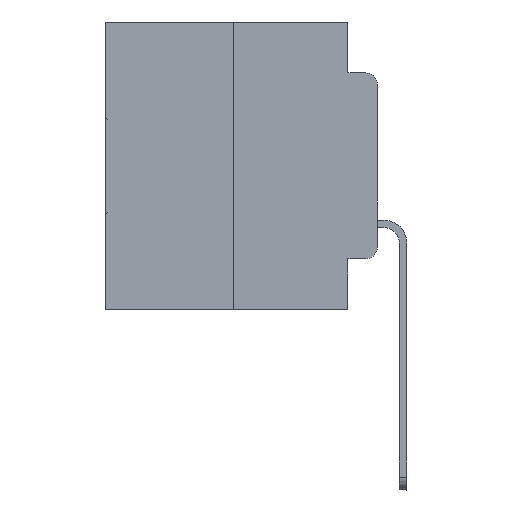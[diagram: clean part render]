
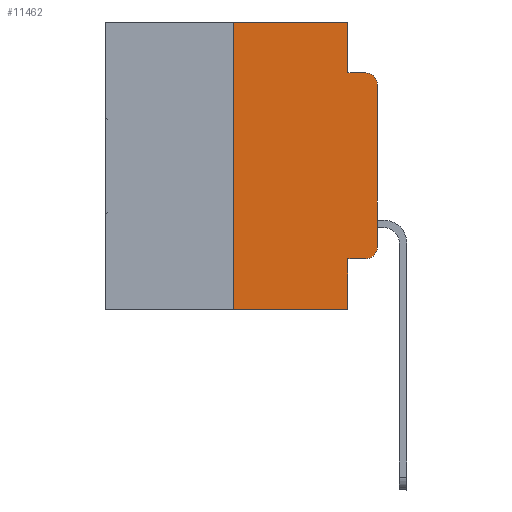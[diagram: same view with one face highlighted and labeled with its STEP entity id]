
A CAD part, left-side view. The second image highlights one B-rep face of the part: STEP entity #11462.
In plain terms, the highlighted planar face has unit normal (-1, 0, 0).
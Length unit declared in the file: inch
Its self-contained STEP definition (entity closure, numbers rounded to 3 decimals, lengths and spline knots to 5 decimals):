
#72 = CARTESIAN_POINT ( 'NONE',  ( 0., 0.051, 0. ) ) ;
#198 = VECTOR ( 'NONE', #6919, 39.37008 ) ;
#233 = CARTESIAN_POINT ( 'NONE',  ( 0., 0.02, -0.1085 ) ) ;
#1229 = VECTOR ( 'NONE', #27164, 39.37008 ) ;
#1791 = LINE ( 'NONE', #11337, #1229 ) ;
#2072 = CARTESIAN_POINT ( 'NONE',  ( 0., 0., 0. ) ) ;
#2083 = VECTOR ( 'NONE', #19083, 39.37008 ) ;
#2942 = LINE ( 'NONE', #9962, #2083 ) ;
#2987 = DIRECTION ( 'NONE',  ( 1., 0., 0. ) ) ;
#3520 = VECTOR ( 'NONE', #17909, 39.37008 ) ;
#4189 = ORIENTED_EDGE ( 'NONE', *, *, #8577, .F. ) ;
#4339 = ORIENTED_EDGE ( 'NONE', *, *, #24047, .F. ) ;
#4835 = LINE ( 'NONE', #24819, #198 ) ;
#5237 = DIRECTION ( 'NONE',  ( 0., 0., -1. ) ) ;
#5364 = VERTEX_POINT ( 'NONE', #17767 ) ;
#5476 = CARTESIAN_POINT ( 'NONE',  ( 0., 0.051, 0. ) ) ;
#6383 = ORIENTED_EDGE ( 'NONE', *, *, #21122, .T. ) ;
#6919 = DIRECTION ( 'NONE',  ( 0., 0., 1. ) ) ;
#8302 = LINE ( 'NONE', #5476, #18983 ) ;
#8577 = EDGE_CURVE ( 'NONE', #17255, #16914, #2942, .T. ) ;
#8653 = DIRECTION ( 'NONE',  ( 0., 0., 1. ) ) ;
#8790 = LINE ( 'NONE', #29236, #3520 ) ;
#8833 = EDGE_CURVE ( 'NONE', #5364, #15069, #4835, .T. ) ;
#9390 = DIRECTION ( 'NONE',  ( 0., 0., -1. ) ) ;
#9706 = EDGE_CURVE ( 'NONE', #5364, #25665, #8790, .T. ) ;
#9962 = CARTESIAN_POINT ( 'NONE',  ( 0., 0.051, -0.0885 ) ) ;
#10247 = CARTESIAN_POINT ( 'NONE',  ( 0., 0., -0.3915 ) ) ;
#11337 = CARTESIAN_POINT ( 'NONE',  ( 0., 0.051, -0.4115 ) ) ;
#11462 = ADVANCED_FACE ( 'NONE', ( #21215 ), #16591, .F. ) ;
#11652 = ORIENTED_EDGE ( 'NONE', *, *, #8833, .F. ) ;
#11819 = ORIENTED_EDGE ( 'NONE', *, *, #9706, .T. ) ;
#12499 = DIRECTION ( 'NONE',  ( 0., 0., -1. ) ) ;
#12764 = CARTESIAN_POINT ( 'NONE',  ( 0., 0.02, -0.0885 ) ) ;
#12994 = LINE ( 'NONE', #2072, #23871 ) ;
#13425 = EDGE_CURVE ( 'NONE', #22376, #20475, #21812, .T. ) ;
#13548 = DIRECTION ( 'NONE',  ( 0., 0., -1. ) ) ;
#13746 = CARTESIAN_POINT ( 'NONE',  ( 0., 0.051, 0. ) ) ;
#14175 = VECTOR ( 'NONE', #9390, 39.37008 ) ;
#15069 = VERTEX_POINT ( 'NONE', #25286 ) ;
#15213 = EDGE_CURVE ( 'NONE', #23148, #17255, #8302, .T. ) ;
#15315 = VECTOR ( 'NONE', #27217, 39.37008 ) ;
#15753 = CARTESIAN_POINT ( 'NONE',  ( 0., 0.473, 0. ) ) ;
#16043 = CARTESIAN_POINT ( 'NONE',  ( 0., 0.051, -0.0885 ) ) ;
#16382 = DIRECTION ( 'NONE',  ( 0., 0., -1. ) ) ;
#16591 = PLANE ( 'NONE',  #19329 ) ;
#16650 = AXIS2_PLACEMENT_3D ( 'NONE', #233, #18336, #16382 ) ;
#16914 = VERTEX_POINT ( 'NONE', #12764 ) ;
#16941 = ORIENTED_EDGE ( 'NONE', *, *, #18420, .F. ) ;
#17255 = VERTEX_POINT ( 'NONE', #16043 ) ;
#17767 = CARTESIAN_POINT ( 'NONE',  ( 0., 0.25, -0.5 ) ) ;
#17909 = DIRECTION ( 'NONE',  ( 0., -1., 0. ) ) ;
#18336 = DIRECTION ( 'NONE',  ( -1., 0., 0. ) ) ;
#18348 = EDGE_LOOP ( 'NONE', ( #28187, #28456, #4189, #22299, #16941, #11652, #11819, #4339, #6383, #21950 ) ) ;
#18420 = EDGE_CURVE ( 'NONE', #15069, #23148, #22760, .T. ) ;
#18475 = CARTESIAN_POINT ( 'NONE',  ( 0., 0.02, -0.3915 ) ) ;
#18634 = CARTESIAN_POINT ( 'NONE',  ( 0., 0.051, -0.5 ) ) ;
#18845 = CARTESIAN_POINT ( 'NONE',  ( 0., 0., -0.1085 ) ) ;
#18983 = VECTOR ( 'NONE', #12499, 39.37008 ) ;
#19007 = VERTEX_POINT ( 'NONE', #18845 ) ;
#19083 = DIRECTION ( 'NONE',  ( 0., -1., 0. ) ) ;
#19129 = CARTESIAN_POINT ( 'NONE',  ( 0., 0.473, 0. ) ) ;
#19329 = AXIS2_PLACEMENT_3D ( 'NONE', #19129, #2987, #5237 ) ;
#19928 = CARTESIAN_POINT ( 'NONE',  ( 0., 0.02, -0.4115 ) ) ;
#20185 = VERTEX_POINT ( 'NONE', #29521 ) ;
#20475 = VERTEX_POINT ( 'NONE', #10247 ) ;
#21122 = EDGE_CURVE ( 'NONE', #20185, #22376, #1791, .T. ) ;
#21215 = FACE_OUTER_BOUND ( 'NONE', #18348, .T. ) ;
#21812 = CIRCLE ( 'NONE', #29428, 0.02 ) ;
#21950 = ORIENTED_EDGE ( 'NONE', *, *, #13425, .T. ) ;
#22299 = ORIENTED_EDGE ( 'NONE', *, *, #15213, .F. ) ;
#22376 = VERTEX_POINT ( 'NONE', #19928 ) ;
#22760 = LINE ( 'NONE', #15753, #15315 ) ;
#22803 = DIRECTION ( 'NONE',  ( -1., 0., 0. ) ) ;
#23148 = VERTEX_POINT ( 'NONE', #72 ) ;
#23871 = VECTOR ( 'NONE', #8653, 39.37008 ) ;
#24047 = EDGE_CURVE ( 'NONE', #20185, #25665, #25052, .T. ) ;
#24819 = CARTESIAN_POINT ( 'NONE',  ( 0., 0.25, 0. ) ) ;
#25052 = LINE ( 'NONE', #13746, #14175 ) ;
#25286 = CARTESIAN_POINT ( 'NONE',  ( 0., 0.25, 0. ) ) ;
#25665 = VERTEX_POINT ( 'NONE', #18634 ) ;
#25678 = EDGE_CURVE ( 'NONE', #19007, #16914, #26165, .T. ) ;
#26165 = CIRCLE ( 'NONE', #16650, 0.02 ) ;
#27164 = DIRECTION ( 'NONE',  ( 0., -1., 0. ) ) ;
#27217 = DIRECTION ( 'NONE',  ( 0., -1., 0. ) ) ;
#28187 = ORIENTED_EDGE ( 'NONE', *, *, #29317, .T. ) ;
#28456 = ORIENTED_EDGE ( 'NONE', *, *, #25678, .T. ) ;
#29236 = CARTESIAN_POINT ( 'NONE',  ( 0., 0.473, -0.5 ) ) ;
#29317 = EDGE_CURVE ( 'NONE', #20475, #19007, #12994, .T. ) ;
#29428 = AXIS2_PLACEMENT_3D ( 'NONE', #18475, #22803, #13548 ) ;
#29521 = CARTESIAN_POINT ( 'NONE',  ( 0., 0.051, -0.4115 ) ) ;
